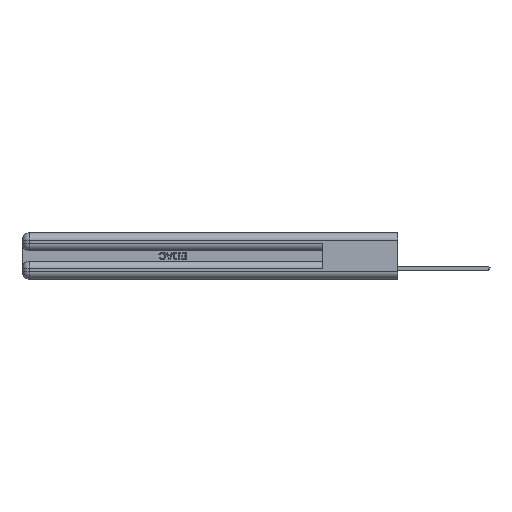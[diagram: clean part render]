
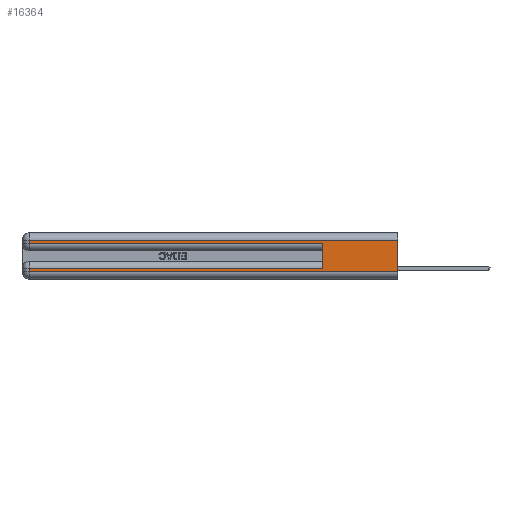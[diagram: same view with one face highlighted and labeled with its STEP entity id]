
A CAD part, left-side view. The second image highlights one B-rep face of the part: STEP entity #16364.
In plain terms, the highlighted planar face has unit normal (-1, 0, 0).
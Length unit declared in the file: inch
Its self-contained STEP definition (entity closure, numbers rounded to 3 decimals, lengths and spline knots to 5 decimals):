
#474 = DIRECTION ( 'NONE',  ( 0., 0., 1. ) ) ;
#3491 = ORIENTED_EDGE ( 'NONE', *, *, #20741, .F. ) ;
#3500 = CARTESIAN_POINT ( 'NONE',  ( 0., 2.94, 0.37 ) ) ;
#3690 = ORIENTED_EDGE ( 'NONE', *, *, #4815, .T. ) ;
#4815 = EDGE_CURVE ( 'NONE', #16368, #10448, #40525, .T. ) ;
#5333 = DIRECTION ( 'NONE',  ( 0., 0., -1. ) ) ;
#5390 = LINE ( 'NONE', #3500, #16484 ) ;
#5885 = VECTOR ( 'NONE', #22430, 39.37008 ) ;
#7575 = ORIENTED_EDGE ( 'NONE', *, *, #39366, .T. ) ;
#9218 = DIRECTION ( 'NONE',  ( 0., 0., -1. ) ) ;
#9644 = LINE ( 'NONE', #19165, #45620 ) ;
#10393 = VERTEX_POINT ( 'NONE', #16104 ) ;
#10442 = EDGE_CURVE ( 'NONE', #12115, #10448, #9644, .T. ) ;
#10448 = VERTEX_POINT ( 'NONE', #19646 ) ;
#11854 = LINE ( 'NONE', #38167, #20310 ) ;
#12115 = VERTEX_POINT ( 'NONE', #32814 ) ;
#12338 = VECTOR ( 'NONE', #33704, 39.37008 ) ;
#13218 = DIRECTION ( 'NONE',  ( 1., 0., 0. ) ) ;
#13223 = CARTESIAN_POINT ( 'NONE',  ( 0., 0., 0.31 ) ) ;
#13772 = VERTEX_POINT ( 'NONE', #25205 ) ;
#14877 = CARTESIAN_POINT ( 'NONE',  ( 0., 0.6, 0.085 ) ) ;
#15455 = ORIENTED_EDGE ( 'NONE', *, *, #37198, .T. ) ;
#16104 = CARTESIAN_POINT ( 'NONE',  ( 0., 2.94, 0.31 ) ) ;
#16241 = LINE ( 'NONE', #29832, #12338 ) ;
#16364 = ADVANCED_FACE ( 'NONE', ( #29341 ), #34197, .F. ) ;
#16368 = VERTEX_POINT ( 'NONE', #23354 ) ;
#16484 = VECTOR ( 'NONE', #42065, 39.37008 ) ;
#17484 = CARTESIAN_POINT ( 'NONE',  ( 0., 0., 0.085 ) ) ;
#19165 = CARTESIAN_POINT ( 'NONE',  ( 0., 0., 0.37 ) ) ;
#19646 = CARTESIAN_POINT ( 'NONE',  ( 0., 0., 0.06 ) ) ;
#20137 = CARTESIAN_POINT ( 'NONE',  ( 0., 0., 0.37 ) ) ;
#20310 = VECTOR ( 'NONE', #474, 39.37008 ) ;
#20741 = EDGE_CURVE ( 'NONE', #30526, #26391, #11854, .T. ) ;
#21637 = ORIENTED_EDGE ( 'NONE', *, *, #30863, .T. ) ;
#22343 = CARTESIAN_POINT ( 'NONE',  ( 0., 0.6, 0.285 ) ) ;
#22430 = DIRECTION ( 'NONE',  ( 0., -1., 0. ) ) ;
#23354 = CARTESIAN_POINT ( 'NONE',  ( 0., 2.94, 0.06 ) ) ;
#24092 = EDGE_LOOP ( 'NONE', ( #31717, #31165, #7575, #21637, #3491, #43047, #15455, #3690 ) ) ;
#24096 = EDGE_CURVE ( 'NONE', #12115, #10393, #24882, .T. ) ;
#24765 = LINE ( 'NONE', #36503, #5885 ) ;
#24882 = LINE ( 'NONE', #13223, #30420 ) ;
#25205 = CARTESIAN_POINT ( 'NONE',  ( 0., 2.94, 0.085 ) ) ;
#26391 = VERTEX_POINT ( 'NONE', #22343 ) ;
#27238 = DIRECTION ( 'NONE',  ( 0., -1., 0. ) ) ;
#28835 = LINE ( 'NONE', #17484, #38240 ) ;
#29341 = FACE_OUTER_BOUND ( 'NONE', #24092, .T. ) ;
#29832 = CARTESIAN_POINT ( 'NONE',  ( 0., 2.94, 0.37 ) ) ;
#30420 = VECTOR ( 'NONE', #38024, 39.37008 ) ;
#30526 = VERTEX_POINT ( 'NONE', #14877 ) ;
#30863 = EDGE_CURVE ( 'NONE', #36336, #26391, #24765, .T. ) ;
#31099 = CARTESIAN_POINT ( 'NONE',  ( 0., 0., 0.06 ) ) ;
#31165 = ORIENTED_EDGE ( 'NONE', *, *, #24096, .T. ) ;
#31215 = VECTOR ( 'NONE', #27238, 39.37008 ) ;
#31717 = ORIENTED_EDGE ( 'NONE', *, *, #10442, .F. ) ;
#32814 = CARTESIAN_POINT ( 'NONE',  ( 0., 0., 0.31 ) ) ;
#33704 = DIRECTION ( 'NONE',  ( 0., 0., -1. ) ) ;
#34197 = PLANE ( 'NONE',  #43002 ) ;
#35453 = EDGE_CURVE ( 'NONE', #30526, #13772, #28835, .T. ) ;
#36336 = VERTEX_POINT ( 'NONE', #39122 ) ;
#36503 = CARTESIAN_POINT ( 'NONE',  ( 0., 0., 0.285 ) ) ;
#37198 = EDGE_CURVE ( 'NONE', #13772, #16368, #5390, .T. ) ;
#38024 = DIRECTION ( 'NONE',  ( 0., 1., 0. ) ) ;
#38167 = CARTESIAN_POINT ( 'NONE',  ( 0., 0.6, 0.145 ) ) ;
#38240 = VECTOR ( 'NONE', #40969, 39.37008 ) ;
#39122 = CARTESIAN_POINT ( 'NONE',  ( 0., 2.94, 0.285 ) ) ;
#39366 = EDGE_CURVE ( 'NONE', #10393, #36336, #16241, .T. ) ;
#40525 = LINE ( 'NONE', #31099, #31215 ) ;
#40969 = DIRECTION ( 'NONE',  ( 0., 1., 0. ) ) ;
#42065 = DIRECTION ( 'NONE',  ( 0., 0., -1. ) ) ;
#43002 = AXIS2_PLACEMENT_3D ( 'NONE', #20137, #13218, #9218 ) ;
#43047 = ORIENTED_EDGE ( 'NONE', *, *, #35453, .T. ) ;
#45620 = VECTOR ( 'NONE', #5333, 39.37008 ) ;
